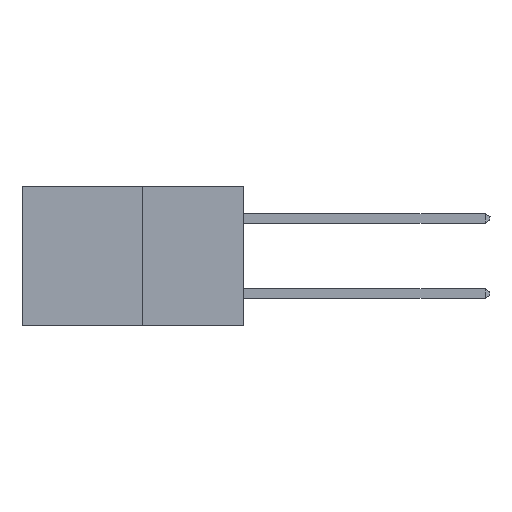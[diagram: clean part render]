
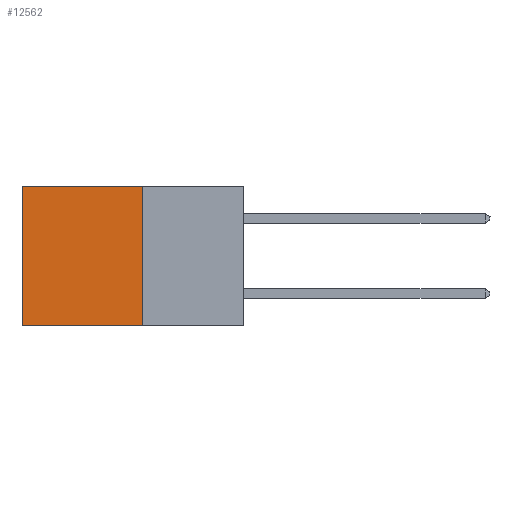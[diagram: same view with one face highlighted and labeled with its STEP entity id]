
A CAD part, left-side view. The second image highlights one B-rep face of the part: STEP entity #12562.
In plain terms, the highlighted planar face has unit normal (-1, 0, 0).
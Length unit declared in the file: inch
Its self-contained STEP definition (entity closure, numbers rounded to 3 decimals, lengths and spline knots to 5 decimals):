
#1216 = DIRECTION ( 'NONE',  ( 0., 0., -1. ) ) ;
#1886 = ORIENTED_EDGE ( 'NONE', *, *, #24173, .T. ) ;
#2016 = VERTEX_POINT ( 'NONE', #4063 ) ;
#2544 = CARTESIAN_POINT ( 'NONE',  ( 0.277, 0.27, 0. ) ) ;
#2889 = FACE_OUTER_BOUND ( 'NONE', #4180, .T. ) ;
#2895 = VERTEX_POINT ( 'NONE', #7525 ) ;
#4063 = CARTESIAN_POINT ( 'NONE',  ( 0.277, 0.59, -0.37 ) ) ;
#4180 = EDGE_LOOP ( 'NONE', ( #22821, #35217, #12331, #1886 ) ) ;
#5303 = CARTESIAN_POINT ( 'NONE',  ( 0.277, 0.27, -0.37 ) ) ;
#7525 = CARTESIAN_POINT ( 'NONE',  ( 0.277, 0.27, -0.37 ) ) ;
#8712 = VECTOR ( 'NONE', #27988, 39.37008 ) ;
#8906 = CARTESIAN_POINT ( 'NONE',  ( 0.277, 0.27, -0.37 ) ) ;
#9376 = DIRECTION ( 'NONE',  ( 0., 0., -1. ) ) ;
#10479 = VECTOR ( 'NONE', #24362, 39.37008 ) ;
#11312 = LINE ( 'NONE', #2544, #10479 ) ;
#12331 = ORIENTED_EDGE ( 'NONE', *, *, #19042, .F. ) ;
#12562 = ADVANCED_FACE ( 'NONE', ( #2889 ), #21598, .F. ) ;
#12732 = CARTESIAN_POINT ( 'NONE',  ( 0.277, 0.27, 0. ) ) ;
#13427 = LINE ( 'NONE', #25638, #14264 ) ;
#14264 = VECTOR ( 'NONE', #9376, 39.37008 ) ;
#15591 = VERTEX_POINT ( 'NONE', #12732 ) ;
#17224 = CARTESIAN_POINT ( 'NONE',  ( 0.277, 0.27, -0.37 ) ) ;
#19042 = EDGE_CURVE ( 'NONE', #15591, #2895, #30360, .T. ) ;
#19118 = EDGE_CURVE ( 'NONE', #32861, #2016, #13427, .T. ) ;
#21598 = PLANE ( 'NONE',  #31864 ) ;
#22821 = ORIENTED_EDGE ( 'NONE', *, *, #19118, .T. ) ;
#24173 = EDGE_CURVE ( 'NONE', #15591, #32861, #11312, .T. ) ;
#24299 = DIRECTION ( 'NONE',  ( 1., 0., 0. ) ) ;
#24362 = DIRECTION ( 'NONE',  ( 0., 1., 0. ) ) ;
#25638 = CARTESIAN_POINT ( 'NONE',  ( 0.277, 0.59, -0.37 ) ) ;
#27085 = LINE ( 'NONE', #8906, #32540 ) ;
#27988 = DIRECTION ( 'NONE',  ( 0., 0., -1. ) ) ;
#29634 = EDGE_CURVE ( 'NONE', #2895, #2016, #27085, .T. ) ;
#29804 = CARTESIAN_POINT ( 'NONE',  ( 0.277, 0.59, 0. ) ) ;
#30360 = LINE ( 'NONE', #17224, #8712 ) ;
#31864 = AXIS2_PLACEMENT_3D ( 'NONE', #5303, #24299, #1216 ) ;
#32540 = VECTOR ( 'NONE', #33339, 39.37008 ) ;
#32861 = VERTEX_POINT ( 'NONE', #29804 ) ;
#33339 = DIRECTION ( 'NONE',  ( 0., 1., 0. ) ) ;
#35217 = ORIENTED_EDGE ( 'NONE', *, *, #29634, .F. ) ;
